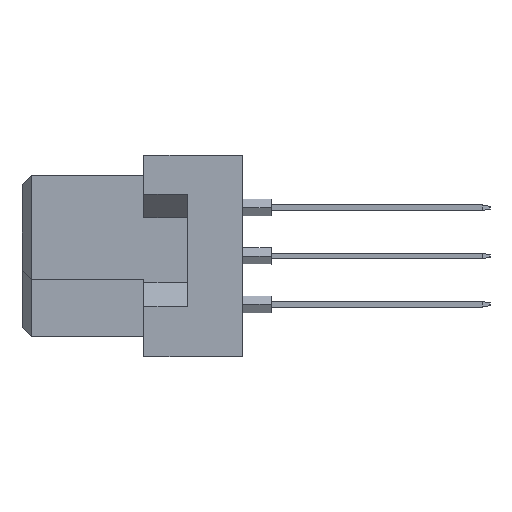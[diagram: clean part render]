
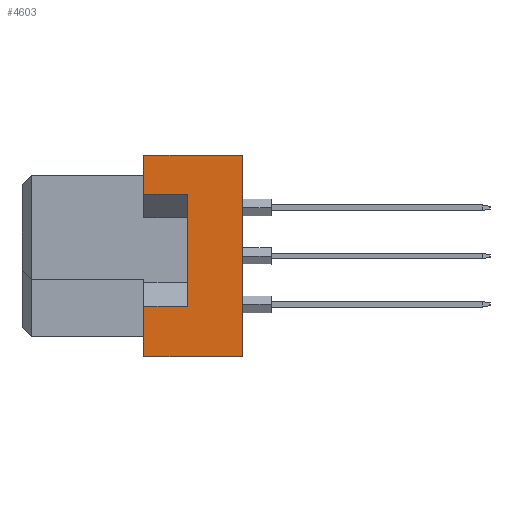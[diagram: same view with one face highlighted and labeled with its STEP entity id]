
A CAD part, left-side view. The second image highlights one B-rep face of the part: STEP entity #4603.
In plain terms, the highlighted planar face has unit normal (-1, 0, 0).
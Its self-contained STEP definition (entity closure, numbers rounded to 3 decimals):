
#280 = LINE ( 'NONE', #22110, #14003 ) ;
#1073 = EDGE_CURVE ( 'NONE', #26152, #13444, #7828, .T. ) ;
#1301 = LINE ( 'NONE', #36628, #3053 ) ;
#1985 = LINE ( 'NONE', #26540, #14504 ) ;
#2424 = VERTEX_POINT ( 'NONE', #24912 ) ;
#3053 = VECTOR ( 'NONE', #17925, 1000. ) ;
#3720 = EDGE_LOOP ( 'NONE', ( #34104, #6574, #16970, #9573, #17575, #13492, #17657, #20350 ) ) ;
#4081 = PLANE ( 'NONE',  #39451 ) ;
#4283 = CARTESIAN_POINT ( 'NONE',  ( -47.5, -11.6, 5.3 ) ) ;
#4603 = ADVANCED_FACE ( 'NONE', ( #19881 ), #4081, .T. ) ;
#5850 = VECTOR ( 'NONE', #10635, 1000. ) ;
#6574 = ORIENTED_EDGE ( 'NONE', *, *, #12223, .F. ) ;
#6702 = DIRECTION ( 'NONE',  ( 0., 0., 1. ) ) ;
#7742 = VERTEX_POINT ( 'NONE', #29452 ) ;
#7828 = LINE ( 'NONE', #14476, #28564 ) ;
#9573 = ORIENTED_EDGE ( 'NONE', *, *, #22340, .T. ) ;
#9768 = DIRECTION ( 'NONE',  ( 0., 0., 1. ) ) ;
#9976 = LINE ( 'NONE', #19126, #38031 ) ;
#10237 = CARTESIAN_POINT ( 'NONE',  ( -47.5, -11.6, 5.3 ) ) ;
#10635 = DIRECTION ( 'NONE',  ( 0., 0., 1. ) ) ;
#12223 = EDGE_CURVE ( 'NONE', #21553, #2424, #37438, .T. ) ;
#13444 = VERTEX_POINT ( 'NONE', #24184 ) ;
#13492 = ORIENTED_EDGE ( 'NONE', *, *, #13811, .F. ) ;
#13811 = EDGE_CURVE ( 'NONE', #13444, #7742, #39094, .T. ) ;
#14003 = VECTOR ( 'NONE', #6702, 1000. ) ;
#14213 = EDGE_CURVE ( 'NONE', #15859, #21553, #1985, .T. ) ;
#14277 = DIRECTION ( 'NONE',  ( 0., 1., 0. ) ) ;
#14476 = CARTESIAN_POINT ( 'NONE',  ( -47.5, -8.7, 3.25 ) ) ;
#14504 = VECTOR ( 'NONE', #26751, 1000. ) ;
#14995 = DIRECTION ( 'NONE',  ( 0., 0., 1. ) ) ;
#15065 = VECTOR ( 'NONE', #14995, 1000. ) ;
#15534 = CARTESIAN_POINT ( 'NONE',  ( -47.5, -11.6, 5.3 ) ) ;
#15859 = VERTEX_POINT ( 'NONE', #32996 ) ;
#16970 = ORIENTED_EDGE ( 'NONE', *, *, #14213, .F. ) ;
#17575 = ORIENTED_EDGE ( 'NONE', *, *, #32331, .T. ) ;
#17657 = ORIENTED_EDGE ( 'NONE', *, *, #1073, .F. ) ;
#17925 = DIRECTION ( 'NONE',  ( 0., 1., 0. ) ) ;
#19126 = CARTESIAN_POINT ( 'NONE',  ( -47.5, -11.6, 5.3 ) ) ;
#19881 = FACE_OUTER_BOUND ( 'NONE', #3720, .T. ) ;
#20350 = ORIENTED_EDGE ( 'NONE', *, *, #26629, .F. ) ;
#21553 = VERTEX_POINT ( 'NONE', #32947 ) ;
#22110 = CARTESIAN_POINT ( 'NONE',  ( -47.5, -8.7, -2.65 ) ) ;
#22340 = EDGE_CURVE ( 'NONE', #15859, #39132, #9976, .T. ) ;
#24184 = CARTESIAN_POINT ( 'NONE',  ( -47.5, -6.4, 3.25 ) ) ;
#24912 = CARTESIAN_POINT ( 'NONE',  ( -47.5, -6.4, -2.65 ) ) ;
#26021 = CARTESIAN_POINT ( 'NONE',  ( -47.5, -6.4, -5.3 ) ) ;
#26152 = VERTEX_POINT ( 'NONE', #39808 ) ;
#26540 = CARTESIAN_POINT ( 'NONE',  ( -47.5, -11.6, -5.3 ) ) ;
#26629 = EDGE_CURVE ( 'NONE', #29224, #26152, #280, .T. ) ;
#26751 = DIRECTION ( 'NONE',  ( 0., 1., 0. ) ) ;
#28217 = VECTOR ( 'NONE', #29756, 1000. ) ;
#28564 = VECTOR ( 'NONE', #14277, 1000. ) ;
#29224 = VERTEX_POINT ( 'NONE', #34650 ) ;
#29443 = DIRECTION ( 'NONE',  ( -1., 0., 0. ) ) ;
#29452 = CARTESIAN_POINT ( 'NONE',  ( -47.5, -6.4, 5.3 ) ) ;
#29756 = DIRECTION ( 'NONE',  ( 0., 1., 0. ) ) ;
#30173 = LINE ( 'NONE', #10237, #28217 ) ;
#32331 = EDGE_CURVE ( 'NONE', #39132, #7742, #30173, .T. ) ;
#32947 = CARTESIAN_POINT ( 'NONE',  ( -47.5, -6.4, -5.3 ) ) ;
#32996 = CARTESIAN_POINT ( 'NONE',  ( -47.5, -11.6, -5.3 ) ) ;
#34104 = ORIENTED_EDGE ( 'NONE', *, *, #35228, .T. ) ;
#34323 = CARTESIAN_POINT ( 'NONE',  ( -47.5, -6.4, -5.3 ) ) ;
#34650 = CARTESIAN_POINT ( 'NONE',  ( -47.5, -8.7, -2.65 ) ) ;
#35228 = EDGE_CURVE ( 'NONE', #29224, #2424, #1301, .T. ) ;
#36628 = CARTESIAN_POINT ( 'NONE',  ( -47.5, -8.7, -2.65 ) ) ;
#37438 = LINE ( 'NONE', #34323, #15065 ) ;
#38031 = VECTOR ( 'NONE', #9768, 1000. ) ;
#39094 = LINE ( 'NONE', #26021, #5850 ) ;
#39132 = VERTEX_POINT ( 'NONE', #15534 ) ;
#39185 = DIRECTION ( 'NONE',  ( 0., 0., 1. ) ) ;
#39451 = AXIS2_PLACEMENT_3D ( 'NONE', #4283, #29443, #39185 ) ;
#39808 = CARTESIAN_POINT ( 'NONE',  ( -47.5, -8.7, 3.25 ) ) ;
